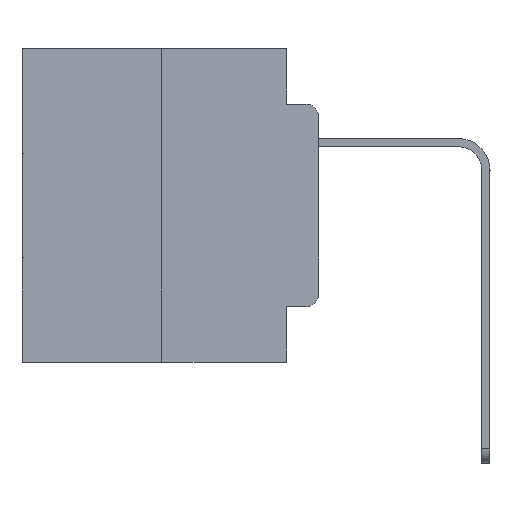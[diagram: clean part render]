
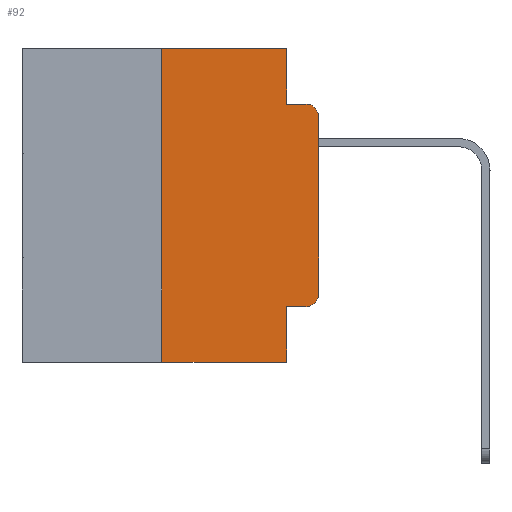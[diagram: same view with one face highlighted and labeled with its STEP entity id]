
A CAD part, left-side view. The second image highlights one B-rep face of the part: STEP entity #92.
In plain terms, the highlighted planar face has unit normal (-1, 0, 0).
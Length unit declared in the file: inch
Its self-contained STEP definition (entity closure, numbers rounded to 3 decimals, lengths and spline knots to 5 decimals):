
#92 = ADVANCED_FACE ( 'NONE', ( #21196 ), #8458, .F. ) ;
#183 = LINE ( 'NONE', #12267, #15426 ) ;
#203 = LINE ( 'NONE', #3488, #26952 ) ;
#429 = DIRECTION ( 'NONE',  ( 0., -1., 0. ) ) ;
#998 = DIRECTION ( 'NONE',  ( 0., 0., -1. ) ) ;
#1064 = AXIS2_PLACEMENT_3D ( 'NONE', #8070, #14245, #7807 ) ;
#1272 = ORIENTED_EDGE ( 'NONE', *, *, #8369, .F. ) ;
#1691 = VECTOR ( 'NONE', #26468, 39.37008 ) ;
#2027 = VERTEX_POINT ( 'NONE', #2362 ) ;
#2362 = CARTESIAN_POINT ( 'NONE',  ( 0., 0.25, -0.5 ) ) ;
#2730 = CARTESIAN_POINT ( 'NONE',  ( 0., 0.473, -0.5 ) ) ;
#2914 = LINE ( 'NONE', #9871, #25213 ) ;
#2994 = ORIENTED_EDGE ( 'NONE', *, *, #5633, .T. ) ;
#3259 = CARTESIAN_POINT ( 'NONE',  ( 0., 0.25, 0. ) ) ;
#3488 = CARTESIAN_POINT ( 'NONE',  ( 0., 0.051, -0.0885 ) ) ;
#3682 = VERTEX_POINT ( 'NONE', #11361 ) ;
#3795 = CARTESIAN_POINT ( 'NONE',  ( 0., 0.051, 0. ) ) ;
#4143 = ORIENTED_EDGE ( 'NONE', *, *, #5081, .T. ) ;
#4475 = CARTESIAN_POINT ( 'NONE',  ( 0., 0.051, -0.4115 ) ) ;
#4515 = EDGE_CURVE ( 'NONE', #5357, #5901, #20992, .T. ) ;
#4929 = VECTOR ( 'NONE', #21026, 39.37008 ) ;
#5081 = EDGE_CURVE ( 'NONE', #22529, #17682, #16053, .T. ) ;
#5297 = CARTESIAN_POINT ( 'NONE',  ( 0., 0.473, 0. ) ) ;
#5357 = VERTEX_POINT ( 'NONE', #4475 ) ;
#5365 = VERTEX_POINT ( 'NONE', #6462 ) ;
#5633 = EDGE_CURVE ( 'NONE', #5357, #22529, #2914, .T. ) ;
#5901 = VERTEX_POINT ( 'NONE', #25514 ) ;
#6023 = DIRECTION ( 'NONE',  ( 0., -1., 0. ) ) ;
#6278 = CARTESIAN_POINT ( 'NONE',  ( 0., 0., -0.3915 ) ) ;
#6374 = EDGE_CURVE ( 'NONE', #5365, #3682, #16380, .T. ) ;
#6443 = DIRECTION ( 'NONE',  ( -1., 0., 0. ) ) ;
#6462 = CARTESIAN_POINT ( 'NONE',  ( 0., 0.051, 0. ) ) ;
#6600 = ORIENTED_EDGE ( 'NONE', *, *, #4515, .F. ) ;
#6827 = ORIENTED_EDGE ( 'NONE', *, *, #6374, .F. ) ;
#7807 = DIRECTION ( 'NONE',  ( 0., 0., -1. ) ) ;
#8070 = CARTESIAN_POINT ( 'NONE',  ( 0., 0.02, -0.3915 ) ) ;
#8235 = EDGE_CURVE ( 'NONE', #20727, #5365, #17664, .T. ) ;
#8244 = AXIS2_PLACEMENT_3D ( 'NONE', #17250, #10729, #25824 ) ;
#8369 = EDGE_CURVE ( 'NONE', #3682, #18652, #203, .T. ) ;
#8458 = PLANE ( 'NONE',  #8244 ) ;
#9333 = ORIENTED_EDGE ( 'NONE', *, *, #8235, .F. ) ;
#9766 = ORIENTED_EDGE ( 'NONE', *, *, #27394, .T. ) ;
#9871 = CARTESIAN_POINT ( 'NONE',  ( 0., 0.051, -0.4115 ) ) ;
#10729 = DIRECTION ( 'NONE',  ( 1., 0., 0. ) ) ;
#11361 = CARTESIAN_POINT ( 'NONE',  ( 0., 0.051, -0.0885 ) ) ;
#11673 = EDGE_CURVE ( 'NONE', #2027, #5901, #25094, .T. ) ;
#11907 = CARTESIAN_POINT ( 'NONE',  ( 0., 0.051, 0. ) ) ;
#11937 = VECTOR ( 'NONE', #20414, 39.37008 ) ;
#12267 = CARTESIAN_POINT ( 'NONE',  ( 0., 0.25, 0. ) ) ;
#12990 = DIRECTION ( 'NONE',  ( 0., 0., -1. ) ) ;
#14245 = DIRECTION ( 'NONE',  ( -1., 0., 0. ) ) ;
#14463 = CARTESIAN_POINT ( 'NONE',  ( 0., 0.02, -0.4115 ) ) ;
#14507 = ORIENTED_EDGE ( 'NONE', *, *, #27418, .F. ) ;
#15426 = VECTOR ( 'NONE', #27357, 39.37008 ) ;
#16053 = CIRCLE ( 'NONE', #1064, 0.02 ) ;
#16220 = CARTESIAN_POINT ( 'NONE',  ( 0., 0.02, -0.0885 ) ) ;
#16380 = LINE ( 'NONE', #11907, #22453 ) ;
#16677 = CARTESIAN_POINT ( 'NONE',  ( 0., 0., 0. ) ) ;
#17231 = CARTESIAN_POINT ( 'NONE',  ( 0., 0.02, -0.1085 ) ) ;
#17250 = CARTESIAN_POINT ( 'NONE',  ( 0., 0.473, 0. ) ) ;
#17516 = ORIENTED_EDGE ( 'NONE', *, *, #24563, .T. ) ;
#17664 = LINE ( 'NONE', #5297, #11937 ) ;
#17682 = VERTEX_POINT ( 'NONE', #6278 ) ;
#18652 = VERTEX_POINT ( 'NONE', #16220 ) ;
#19253 = EDGE_LOOP ( 'NONE', ( #9766, #17516, #1272, #6827, #9333, #14507, #24438, #6600, #2994, #4143 ) ) ;
#20147 = CIRCLE ( 'NONE', #27736, 0.02 ) ;
#20414 = DIRECTION ( 'NONE',  ( 0., -1., 0. ) ) ;
#20714 = DIRECTION ( 'NONE',  ( 0., -1., 0. ) ) ;
#20727 = VERTEX_POINT ( 'NONE', #3259 ) ;
#20781 = VERTEX_POINT ( 'NONE', #24709 ) ;
#20992 = LINE ( 'NONE', #3795, #1691 ) ;
#21026 = DIRECTION ( 'NONE',  ( 0., 0., 1. ) ) ;
#21196 = FACE_OUTER_BOUND ( 'NONE', #19253, .T. ) ;
#21833 = LINE ( 'NONE', #16677, #4929 ) ;
#22453 = VECTOR ( 'NONE', #998, 39.37008 ) ;
#22529 = VERTEX_POINT ( 'NONE', #14463 ) ;
#23408 = VECTOR ( 'NONE', #429, 39.37008 ) ;
#24438 = ORIENTED_EDGE ( 'NONE', *, *, #11673, .T. ) ;
#24563 = EDGE_CURVE ( 'NONE', #20781, #18652, #20147, .T. ) ;
#24709 = CARTESIAN_POINT ( 'NONE',  ( 0., 0., -0.1085 ) ) ;
#25094 = LINE ( 'NONE', #2730, #23408 ) ;
#25213 = VECTOR ( 'NONE', #20714, 39.37008 ) ;
#25514 = CARTESIAN_POINT ( 'NONE',  ( 0., 0.051, -0.5 ) ) ;
#25824 = DIRECTION ( 'NONE',  ( 0., 0., -1. ) ) ;
#26468 = DIRECTION ( 'NONE',  ( 0., 0., -1. ) ) ;
#26952 = VECTOR ( 'NONE', #6023, 39.37008 ) ;
#27357 = DIRECTION ( 'NONE',  ( 0., 0., 1. ) ) ;
#27394 = EDGE_CURVE ( 'NONE', #17682, #20781, #21833, .T. ) ;
#27418 = EDGE_CURVE ( 'NONE', #2027, #20727, #183, .T. ) ;
#27736 = AXIS2_PLACEMENT_3D ( 'NONE', #17231, #6443, #12990 ) ;
